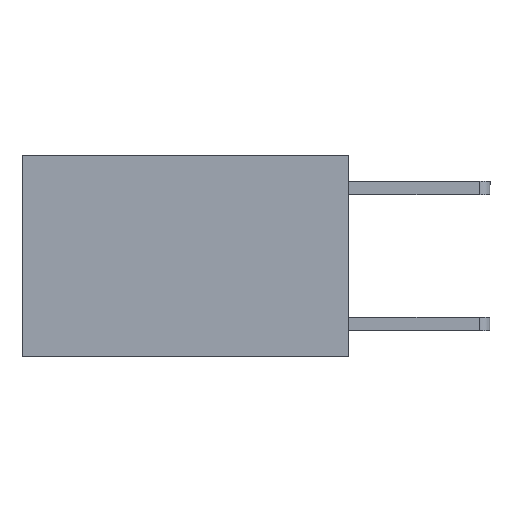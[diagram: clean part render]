
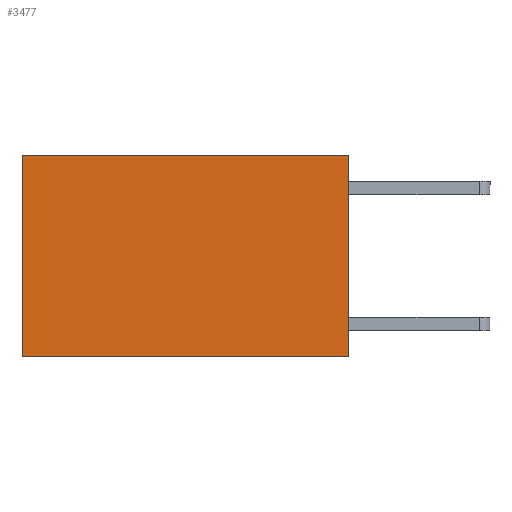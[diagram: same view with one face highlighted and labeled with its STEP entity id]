
A CAD part, left-side view. The second image highlights one B-rep face of the part: STEP entity #3477.
In plain terms, the highlighted planar face has unit normal (-1, 0, 0).
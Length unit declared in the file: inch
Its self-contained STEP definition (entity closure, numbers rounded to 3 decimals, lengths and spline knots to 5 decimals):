
#7 = PLANE ( 'NONE',  #6789 ) ;
#227 = VECTOR ( 'NONE', #3317, 39.37008 ) ;
#819 = VERTEX_POINT ( 'NONE', #2470 ) ;
#849 = ORIENTED_EDGE ( 'NONE', *, *, #5422, .F. ) ;
#1181 = LINE ( 'NONE', #1809, #227 ) ;
#1317 = DIRECTION ( 'NONE',  ( 1., 0., 0. ) ) ;
#1381 = VECTOR ( 'NONE', #6076, 39.37008 ) ;
#1609 = VECTOR ( 'NONE', #2591, 39.37008 ) ;
#1809 = CARTESIAN_POINT ( 'NONE',  ( 0.2625, 0.6, 0. ) ) ;
#1889 = DIRECTION ( 'NONE',  ( 0., 0., -1. ) ) ;
#2470 = CARTESIAN_POINT ( 'NONE',  ( 0.2625, 0., 0. ) ) ;
#2591 = DIRECTION ( 'NONE',  ( 0., 1., 0. ) ) ;
#2629 = CARTESIAN_POINT ( 'NONE',  ( 0.2625, 0.6, -0.37 ) ) ;
#3317 = DIRECTION ( 'NONE',  ( 0., 0., -1. ) ) ;
#3477 = ADVANCED_FACE ( 'NONE', ( #7564 ), #7, .F. ) ;
#3900 = EDGE_CURVE ( 'NONE', #819, #4856, #7526, .T. ) ;
#4140 = EDGE_LOOP ( 'NONE', ( #4787, #849, #6416, #5025 ) ) ;
#4787 = ORIENTED_EDGE ( 'NONE', *, *, #5378, .T. ) ;
#4856 = VERTEX_POINT ( 'NONE', #5903 ) ;
#5025 = ORIENTED_EDGE ( 'NONE', *, *, #3900, .T. ) ;
#5237 = CARTESIAN_POINT ( 'NONE',  ( 0.2625, 0., 0. ) ) ;
#5360 = DIRECTION ( 'NONE',  ( 0., 0., -1. ) ) ;
#5378 = EDGE_CURVE ( 'NONE', #4856, #8613, #1181, .T. ) ;
#5422 = EDGE_CURVE ( 'NONE', #7141, #8613, #8784, .T. ) ;
#5491 = CARTESIAN_POINT ( 'NONE',  ( 0.2625, 0., 0. ) ) ;
#5903 = CARTESIAN_POINT ( 'NONE',  ( 0.2625, 0.6, 0. ) ) ;
#5983 = CARTESIAN_POINT ( 'NONE',  ( 0.2625, 0., -0.37 ) ) ;
#6076 = DIRECTION ( 'NONE',  ( 0., 1., 0. ) ) ;
#6416 = ORIENTED_EDGE ( 'NONE', *, *, #8128, .F. ) ;
#6789 = AXIS2_PLACEMENT_3D ( 'NONE', #8155, #1317, #5360 ) ;
#6860 = CARTESIAN_POINT ( 'NONE',  ( 0.2625, 0., -0.37 ) ) ;
#7141 = VERTEX_POINT ( 'NONE', #6860 ) ;
#7526 = LINE ( 'NONE', #5491, #1609 ) ;
#7564 = FACE_OUTER_BOUND ( 'NONE', #4140, .T. ) ;
#8128 = EDGE_CURVE ( 'NONE', #819, #7141, #8813, .T. ) ;
#8155 = CARTESIAN_POINT ( 'NONE',  ( 0.2625, 0., 0. ) ) ;
#8494 = VECTOR ( 'NONE', #1889, 39.37008 ) ;
#8613 = VERTEX_POINT ( 'NONE', #2629 ) ;
#8784 = LINE ( 'NONE', #5983, #1381 ) ;
#8813 = LINE ( 'NONE', #5237, #8494 ) ;
